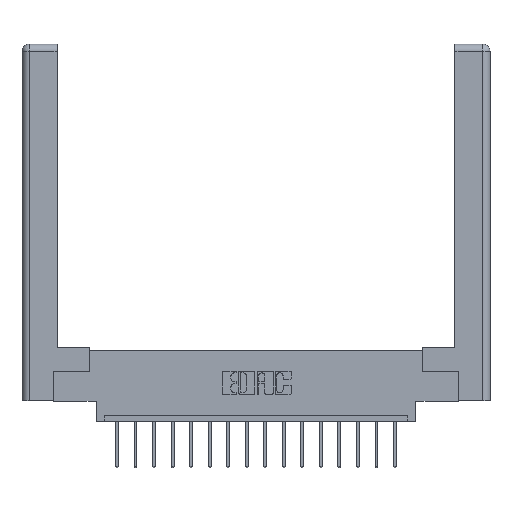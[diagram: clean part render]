
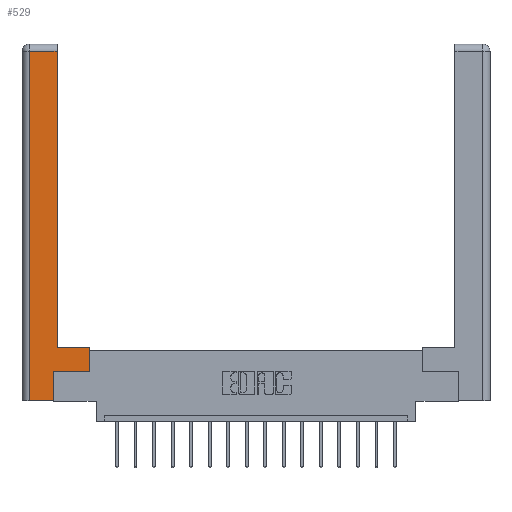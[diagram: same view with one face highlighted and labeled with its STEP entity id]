
A CAD part, top view. The second image highlights one B-rep face of the part: STEP entity #529.
In plain terms, the highlighted planar face has unit normal (0, 0, 1).
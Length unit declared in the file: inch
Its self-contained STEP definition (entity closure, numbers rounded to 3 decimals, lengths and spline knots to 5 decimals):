
#198 = ORIENTED_EDGE ( 'NONE', *, *, #8034, .T. ) ;
#529 = ADVANCED_FACE ( 'NONE', ( #2676 ), #2679, .F. ) ;
#768 = CARTESIAN_POINT ( 'NONE',  ( 0.265, 0.245, 0. ) ) ;
#1828 = ORIENTED_EDGE ( 'NONE', *, *, #11143, .T. ) ;
#2327 = AXIS2_PLACEMENT_3D ( 'NONE', #16566, #16733, #8397 ) ;
#2334 = EDGE_CURVE ( 'NONE', #6785, #12586, #5654, .T. ) ;
#2579 = VECTOR ( 'NONE', #3117, 39.37008 ) ;
#2598 = CARTESIAN_POINT ( 'NONE',  ( 0.295, 0.45, 0. ) ) ;
#2676 = FACE_OUTER_BOUND ( 'NONE', #7709, .T. ) ;
#2679 = PLANE ( 'NONE',  #2327 ) ;
#2883 = CARTESIAN_POINT ( 'NONE',  ( 0.295, 2.94, 0. ) ) ;
#2918 = CARTESIAN_POINT ( 'NONE',  ( 0.565, 0.245, 0. ) ) ;
#2976 = DIRECTION ( 'NONE',  ( 1., 0., 0. ) ) ;
#3117 = DIRECTION ( 'NONE',  ( 0., 1., 0. ) ) ;
#3578 = DIRECTION ( 'NONE',  ( -1., 0., 0. ) ) ;
#5114 = CARTESIAN_POINT ( 'NONE',  ( 0.265, 0., 0. ) ) ;
#5432 = LINE ( 'NONE', #16655, #8026 ) ;
#5654 = LINE ( 'NONE', #14523, #12201 ) ;
#5946 = DIRECTION ( 'NONE',  ( 0., 1., 0. ) ) ;
#6074 = VERTEX_POINT ( 'NONE', #5114 ) ;
#6235 = ORIENTED_EDGE ( 'NONE', *, *, #16888, .T. ) ;
#6611 = VECTOR ( 'NONE', #2976, 39.37008 ) ;
#6703 = VERTEX_POINT ( 'NONE', #18047 ) ;
#6785 = VERTEX_POINT ( 'NONE', #9769 ) ;
#6900 = EDGE_CURVE ( 'NONE', #6074, #7682, #8250, .T. ) ;
#6999 = VERTEX_POINT ( 'NONE', #10366 ) ;
#7230 = CARTESIAN_POINT ( 'NONE',  ( 0.265, 0., 0. ) ) ;
#7682 = VERTEX_POINT ( 'NONE', #768 ) ;
#7709 = EDGE_LOOP ( 'NONE', ( #15506, #6235, #9622, #13811, #17977, #10067, #1828, #198 ) ) ;
#8026 = VECTOR ( 'NONE', #15213, 39.37008 ) ;
#8034 = EDGE_CURVE ( 'NONE', #6703, #6785, #11261, .T. ) ;
#8250 = LINE ( 'NONE', #11472, #2579 ) ;
#8296 = CARTESIAN_POINT ( 'NONE',  ( 0.0615, 0., 0. ) ) ;
#8397 = DIRECTION ( 'NONE',  ( -1., 0., 0. ) ) ;
#8649 = CARTESIAN_POINT ( 'NONE',  ( 0.0615, 2.94, 0. ) ) ;
#9126 = CARTESIAN_POINT ( 'NONE',  ( 0.0615, 2.94, 0. ) ) ;
#9622 = ORIENTED_EDGE ( 'NONE', *, *, #13401, .T. ) ;
#9769 = CARTESIAN_POINT ( 'NONE',  ( 0.295, 0.45, 0. ) ) ;
#10067 = ORIENTED_EDGE ( 'NONE', *, *, #10594, .T. ) ;
#10099 = LINE ( 'NONE', #2918, #6611 ) ;
#10366 = CARTESIAN_POINT ( 'NONE',  ( 0.565, 0.245, 0. ) ) ;
#10594 = EDGE_CURVE ( 'NONE', #7682, #6999, #10099, .T. ) ;
#10714 = CARTESIAN_POINT ( 'NONE',  ( 0.0615, 0., 0. ) ) ;
#11081 = DIRECTION ( 'NONE',  ( -1., 0., 0. ) ) ;
#11143 = EDGE_CURVE ( 'NONE', #6999, #6703, #5432, .T. ) ;
#11261 = LINE ( 'NONE', #2598, #17804 ) ;
#11472 = CARTESIAN_POINT ( 'NONE',  ( 0.265, 0.245, 0. ) ) ;
#11631 = VECTOR ( 'NONE', #3578, 39.37008 ) ;
#12001 = LINE ( 'NONE', #8296, #17646 ) ;
#12201 = VECTOR ( 'NONE', #5946, 39.37008 ) ;
#12586 = VERTEX_POINT ( 'NONE', #2883 ) ;
#12710 = DIRECTION ( 'NONE',  ( 1., 0., 0. ) ) ;
#13398 = VERTEX_POINT ( 'NONE', #8649 ) ;
#13401 = EDGE_CURVE ( 'NONE', #13398, #14243, #12001, .T. ) ;
#13811 = ORIENTED_EDGE ( 'NONE', *, *, #17811, .T. ) ;
#14243 = VERTEX_POINT ( 'NONE', #10714 ) ;
#14315 = DIRECTION ( 'NONE',  ( 0., -1., 0. ) ) ;
#14523 = CARTESIAN_POINT ( 'NONE',  ( 0.295, 3., 0. ) ) ;
#14866 = VECTOR ( 'NONE', #12710, 39.37008 ) ;
#15213 = DIRECTION ( 'NONE',  ( 0., 1., 0. ) ) ;
#15506 = ORIENTED_EDGE ( 'NONE', *, *, #2334, .T. ) ;
#16193 = LINE ( 'NONE', #9126, #11631 ) ;
#16378 = LINE ( 'NONE', #7230, #14866 ) ;
#16566 = CARTESIAN_POINT ( 'NONE',  ( 0., 0., 0. ) ) ;
#16655 = CARTESIAN_POINT ( 'NONE',  ( 0.565, 0.45, 0. ) ) ;
#16733 = DIRECTION ( 'NONE',  ( 0., 0., -1. ) ) ;
#16888 = EDGE_CURVE ( 'NONE', #12586, #13398, #16193, .T. ) ;
#17646 = VECTOR ( 'NONE', #14315, 39.37008 ) ;
#17804 = VECTOR ( 'NONE', #11081, 39.37008 ) ;
#17811 = EDGE_CURVE ( 'NONE', #14243, #6074, #16378, .T. ) ;
#17977 = ORIENTED_EDGE ( 'NONE', *, *, #6900, .T. ) ;
#18047 = CARTESIAN_POINT ( 'NONE',  ( 0.565, 0.45, 0. ) ) ;
